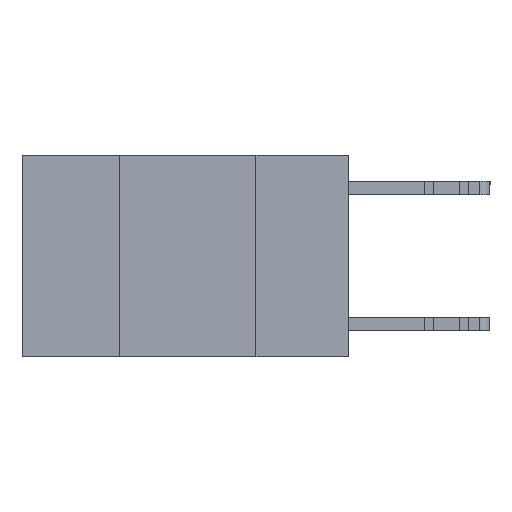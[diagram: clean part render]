
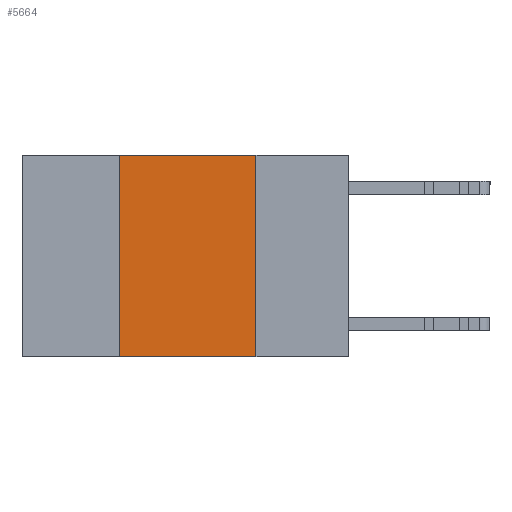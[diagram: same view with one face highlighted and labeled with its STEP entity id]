
A CAD part, left-side view. The second image highlights one B-rep face of the part: STEP entity #5664.
In plain terms, the highlighted planar face has unit normal (-1, 0, 0).
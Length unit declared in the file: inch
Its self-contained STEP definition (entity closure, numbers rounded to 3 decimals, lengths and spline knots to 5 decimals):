
#360 = LINE ( 'NONE', #18329, #12072 ) ;
#422 = CARTESIAN_POINT ( 'NONE',  ( 0., 0.6, 0. ) ) ;
#1923 = VECTOR ( 'NONE', #14497, 39.37008 ) ;
#2638 = PLANE ( 'NONE',  #23099 ) ;
#3872 = VERTEX_POINT ( 'NONE', #21285 ) ;
#3969 = EDGE_CURVE ( 'NONE', #3872, #22816, #7466, .T. ) ;
#4976 = DIRECTION ( 'NONE',  ( 0., 0., -1. ) ) ;
#5369 = EDGE_CURVE ( 'NONE', #21174, #3872, #10010, .T. ) ;
#5664 = ADVANCED_FACE ( 'NONE', ( #20610 ), #2638, .F. ) ;
#5674 = ORIENTED_EDGE ( 'NONE', *, *, #19045, .F. ) ;
#7355 = DIRECTION ( 'NONE',  ( 1., 0., 0. ) ) ;
#7466 = LINE ( 'NONE', #12297, #1923 ) ;
#7610 = ORIENTED_EDGE ( 'NONE', *, *, #19367, .T. ) ;
#8245 = DIRECTION ( 'NONE',  ( 0., -1., 0. ) ) ;
#8846 = ORIENTED_EDGE ( 'NONE', *, *, #3969, .F. ) ;
#10010 = LINE ( 'NONE', #14853, #13212 ) ;
#10460 = EDGE_LOOP ( 'NONE', ( #8846, #18886, #5674, #7610 ) ) ;
#10935 = DIRECTION ( 'NONE',  ( 0., -1., 0. ) ) ;
#10942 = CARTESIAN_POINT ( 'NONE',  ( 0., 0.42, -0.37 ) ) ;
#12072 = VECTOR ( 'NONE', #26862, 39.37008 ) ;
#12297 = CARTESIAN_POINT ( 'NONE',  ( 0., 0.17, 0. ) ) ;
#13212 = VECTOR ( 'NONE', #8245, 39.37008 ) ;
#14052 = LINE ( 'NONE', #19627, #14409 ) ;
#14409 = VECTOR ( 'NONE', #10935, 39.37008 ) ;
#14497 = DIRECTION ( 'NONE',  ( 0., 0., -1. ) ) ;
#14722 = CARTESIAN_POINT ( 'NONE',  ( 0., 0.42, 0. ) ) ;
#14853 = CARTESIAN_POINT ( 'NONE',  ( 0., 0.6, 0. ) ) ;
#18329 = CARTESIAN_POINT ( 'NONE',  ( 0., 0.42, 0. ) ) ;
#18886 = ORIENTED_EDGE ( 'NONE', *, *, #5369, .F. ) ;
#19045 = EDGE_CURVE ( 'NONE', #28309, #21174, #360, .T. ) ;
#19367 = EDGE_CURVE ( 'NONE', #28309, #22816, #14052, .T. ) ;
#19627 = CARTESIAN_POINT ( 'NONE',  ( 0., 0.6, -0.37 ) ) ;
#20610 = FACE_OUTER_BOUND ( 'NONE', #10460, .T. ) ;
#21174 = VERTEX_POINT ( 'NONE', #14722 ) ;
#21285 = CARTESIAN_POINT ( 'NONE',  ( 0., 0.17, 0. ) ) ;
#22816 = VERTEX_POINT ( 'NONE', #26834 ) ;
#23099 = AXIS2_PLACEMENT_3D ( 'NONE', #422, #7355, #4976 ) ;
#26834 = CARTESIAN_POINT ( 'NONE',  ( 0., 0.17, -0.37 ) ) ;
#26862 = DIRECTION ( 'NONE',  ( 0., 0., 1. ) ) ;
#28309 = VERTEX_POINT ( 'NONE', #10942 ) ;
